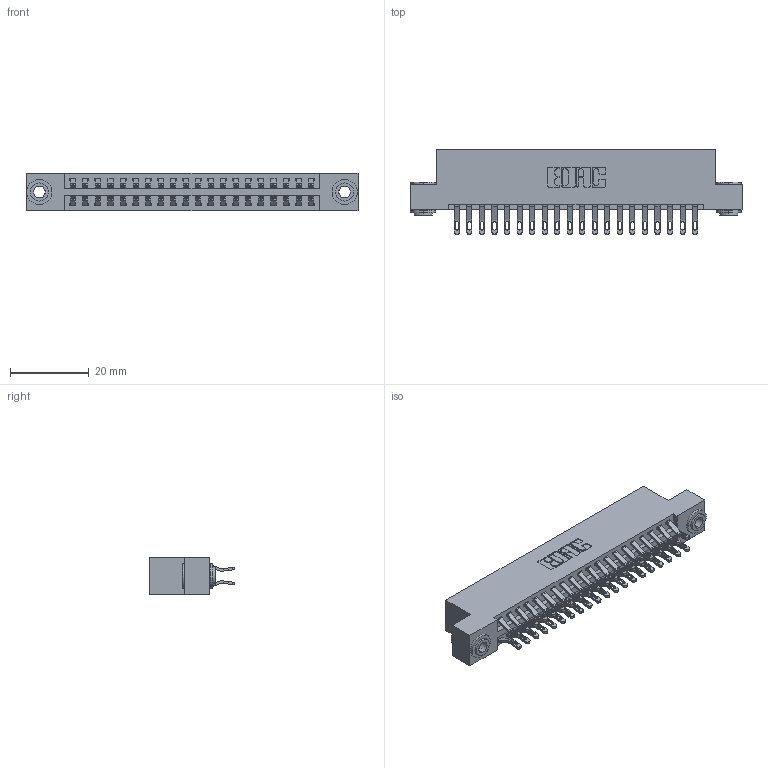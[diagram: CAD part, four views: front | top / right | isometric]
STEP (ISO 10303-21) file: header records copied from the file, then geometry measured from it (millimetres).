
FILE_DESCRIPTION (( 'STEP AP203' ), '1' );
FILE_NAME ('346-040-555-203.STEP', '2022-05-20T02:21:54', ( '' ), ( '' ), 'SwSTEP 2.0', 'SolidWorks 2020', '' );
FILE_SCHEMA (( 'CONFIG_CONTROL_DESIGN' ));
Length unit declared in the file: inch
Products named in the file (4): 345-292-001_555 Tail; 346-040-555-203; 345-250-002_345-250-002-102; 346 Part_Flush Mounting Lugs - 0.156 Dia-TH
Assembly tree (43 placements, depth 2):
  346-040-555-203
    346 Part_Flush Mounting Lugs - 0.156 Dia-TH
    345-292-001_555 Tail  x40
    345-250-002_345-250-002-102  x2
Bounding box: 84.07 x 21.46 x 9.4 mm (x, y, z)
Volume: 8144.7 mm3; surface area: 11512 mm2
Topology: 43 solids, 43 shells, 2494 faces, 7761 edges, 5170 vertices
Faces by surface type: plane 1420, cylinder 1066, cone 8
Entity records: 17406 total; most frequent: CARTESIAN_POINT 2915, ORIENTED_EDGE 2810, DIRECTION 2619, EDGE_CURVE 1405, VECTOR 1149, LINE 1149, VERTEX_POINT 934, AXIS2_PLACEMENT_3D 735
